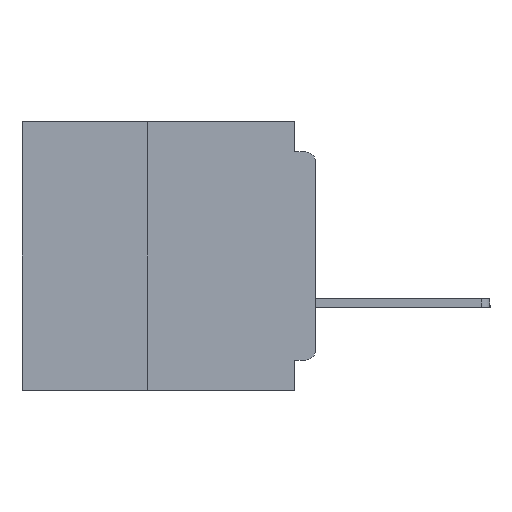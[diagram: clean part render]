
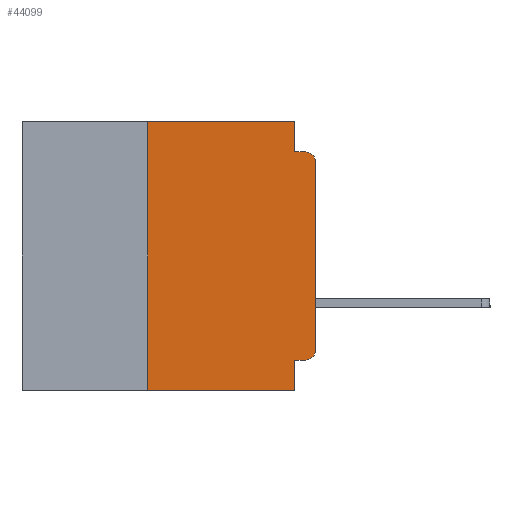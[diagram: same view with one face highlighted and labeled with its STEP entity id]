
A CAD part, left-side view. The second image highlights one B-rep face of the part: STEP entity #44099.
In plain terms, the highlighted planar face has unit normal (-1, 0, 0).
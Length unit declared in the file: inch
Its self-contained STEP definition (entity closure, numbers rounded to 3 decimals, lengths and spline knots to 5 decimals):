
#526 = LINE ( 'NONE', #22657, #59497 ) ;
#994 = VERTEX_POINT ( 'NONE', #20678 ) ;
#1742 = CARTESIAN_POINT ( 'NONE',  ( 0., 0.437, 0. ) ) ;
#2908 = EDGE_CURVE ( 'NONE', #36911, #27660, #33118, .T. ) ;
#2958 = LINE ( 'NONE', #53123, #18271 ) ;
#3637 = CARTESIAN_POINT ( 'NONE',  ( 0., 0.031, -0.4 ) ) ;
#4300 = CARTESIAN_POINT ( 'NONE',  ( 0., 0.031, 0. ) ) ;
#6065 = ORIENTED_EDGE ( 'NONE', *, *, #49792, .T. ) ;
#6183 = DIRECTION ( 'NONE',  ( 0., 0., -1. ) ) ;
#6405 = CIRCLE ( 'NONE', #38215, 0.015 ) ;
#6409 = PLANE ( 'NONE',  #52986 ) ;
#6523 = FACE_OUTER_BOUND ( 'NONE', #28270, .T. ) ;
#8288 = VECTOR ( 'NONE', #56010, 39.37008 ) ;
#8735 = DIRECTION ( 'NONE',  ( 0., -1., 0. ) ) ;
#8841 = LINE ( 'NONE', #49030, #32197 ) ;
#11990 = ORIENTED_EDGE ( 'NONE', *, *, #19523, .T. ) ;
#13692 = LINE ( 'NONE', #60333, #47957 ) ;
#14111 = DIRECTION ( 'NONE',  ( -1., 0., 0. ) ) ;
#14444 = VERTEX_POINT ( 'NONE', #48058 ) ;
#14611 = AXIS2_PLACEMENT_3D ( 'NONE', #42071, #14111, #46723 ) ;
#15791 = DIRECTION ( 'NONE',  ( 0., 0., -1. ) ) ;
#16769 = EDGE_CURVE ( 'NONE', #31690, #25327, #13692, .T. ) ;
#17154 = ORIENTED_EDGE ( 'NONE', *, *, #16769, .F. ) ;
#17900 = ORIENTED_EDGE ( 'NONE', *, *, #31625, .T. ) ;
#18271 = VECTOR ( 'NONE', #57808, 39.37008 ) ;
#18971 = VECTOR ( 'NONE', #6183, 39.37008 ) ;
#19523 = EDGE_CURVE ( 'NONE', #44456, #994, #24437, .T. ) ;
#20619 = DIRECTION ( 'NONE',  ( 0., 0., -1. ) ) ;
#20678 = CARTESIAN_POINT ( 'NONE',  ( 0., 0., -0.34 ) ) ;
#21519 = CARTESIAN_POINT ( 'NONE',  ( 0., 0., -0.355 ) ) ;
#21760 = LINE ( 'NONE', #25354, #57418 ) ;
#22657 = CARTESIAN_POINT ( 'NONE',  ( 0., 0., -0.045 ) ) ;
#22922 = VECTOR ( 'NONE', #58714, 39.37008 ) ;
#22996 = DIRECTION ( 'NONE',  ( 0., -1., 0. ) ) ;
#24437 = CIRCLE ( 'NONE', #14611, 0.015 ) ;
#24938 = EDGE_CURVE ( 'NONE', #25327, #28747, #31392, .T. ) ;
#25327 = VERTEX_POINT ( 'NONE', #4300 ) ;
#25354 = CARTESIAN_POINT ( 'NONE',  ( 0., 0.031, -0.4 ) ) ;
#25962 = DIRECTION ( 'NONE',  ( -1., 0., 0. ) ) ;
#27660 = VERTEX_POINT ( 'NONE', #3637 ) ;
#28270 = EDGE_LOOP ( 'NONE', ( #6065, #17900, #44654, #50144, #17154, #36712, #51407, #57345, #50468, #11990 ) ) ;
#28747 = VERTEX_POINT ( 'NONE', #30287 ) ;
#30287 = CARTESIAN_POINT ( 'NONE',  ( 0., 0.031, -0.045 ) ) ;
#31392 = LINE ( 'NONE', #38831, #18971 ) ;
#31576 = EDGE_CURVE ( 'NONE', #14444, #27660, #21760, .T. ) ;
#31625 = EDGE_CURVE ( 'NONE', #54610, #39142, #6405, .T. ) ;
#31690 = VERTEX_POINT ( 'NONE', #49705 ) ;
#32197 = VECTOR ( 'NONE', #48824, 39.37008 ) ;
#32480 = CARTESIAN_POINT ( 'NONE',  ( 0., 0.015, -0.045 ) ) ;
#33118 = LINE ( 'NONE', #42016, #8288 ) ;
#36712 = ORIENTED_EDGE ( 'NONE', *, *, #50391, .F. ) ;
#36911 = VERTEX_POINT ( 'NONE', #51762 ) ;
#38215 = AXIS2_PLACEMENT_3D ( 'NONE', #53772, #25962, #58422 ) ;
#38831 = CARTESIAN_POINT ( 'NONE',  ( 0., 0.031, 0. ) ) ;
#39142 = VERTEX_POINT ( 'NONE', #32480 ) ;
#42016 = CARTESIAN_POINT ( 'NONE',  ( 0., 0.437, -0.4 ) ) ;
#42071 = CARTESIAN_POINT ( 'NONE',  ( 0., 0.015, -0.34 ) ) ;
#43757 = DIRECTION ( 'NONE',  ( 1., 0., 0. ) ) ;
#44099 = ADVANCED_FACE ( 'NONE', ( #6523 ), #6409, .F. ) ;
#44456 = VERTEX_POINT ( 'NONE', #55244 ) ;
#44654 = ORIENTED_EDGE ( 'NONE', *, *, #46126, .F. ) ;
#45055 = CARTESIAN_POINT ( 'NONE',  ( 0., 0., -0.06 ) ) ;
#46126 = EDGE_CURVE ( 'NONE', #28747, #39142, #526, .T. ) ;
#46723 = DIRECTION ( 'NONE',  ( 0., 0., -1. ) ) ;
#47957 = VECTOR ( 'NONE', #22996, 39.37008 ) ;
#48058 = CARTESIAN_POINT ( 'NONE',  ( 0., 0.031, -0.355 ) ) ;
#48064 = EDGE_CURVE ( 'NONE', #44456, #14444, #50579, .T. ) ;
#48824 = DIRECTION ( 'NONE',  ( 0., 0., 1. ) ) ;
#49030 = CARTESIAN_POINT ( 'NONE',  ( 0., 0., 0. ) ) ;
#49705 = CARTESIAN_POINT ( 'NONE',  ( 0., 0.25, 0. ) ) ;
#49792 = EDGE_CURVE ( 'NONE', #994, #54610, #8841, .T. ) ;
#50144 = ORIENTED_EDGE ( 'NONE', *, *, #24938, .F. ) ;
#50391 = EDGE_CURVE ( 'NONE', #36911, #31690, #2958, .T. ) ;
#50468 = ORIENTED_EDGE ( 'NONE', *, *, #48064, .F. ) ;
#50579 = LINE ( 'NONE', #21519, #22922 ) ;
#51407 = ORIENTED_EDGE ( 'NONE', *, *, #2908, .T. ) ;
#51762 = CARTESIAN_POINT ( 'NONE',  ( 0., 0.25, -0.4 ) ) ;
#52986 = AXIS2_PLACEMENT_3D ( 'NONE', #1742, #43757, #15791 ) ;
#53123 = CARTESIAN_POINT ( 'NONE',  ( 0., 0.25, -0.4 ) ) ;
#53772 = CARTESIAN_POINT ( 'NONE',  ( 0., 0.015, -0.06 ) ) ;
#54610 = VERTEX_POINT ( 'NONE', #45055 ) ;
#55244 = CARTESIAN_POINT ( 'NONE',  ( 0., 0.015, -0.355 ) ) ;
#56010 = DIRECTION ( 'NONE',  ( 0., -1., 0. ) ) ;
#57345 = ORIENTED_EDGE ( 'NONE', *, *, #31576, .F. ) ;
#57418 = VECTOR ( 'NONE', #20619, 39.37008 ) ;
#57808 = DIRECTION ( 'NONE',  ( 0., 0., 1. ) ) ;
#58422 = DIRECTION ( 'NONE',  ( 0., 0., -1. ) ) ;
#58714 = DIRECTION ( 'NONE',  ( 0., 1., 0. ) ) ;
#59497 = VECTOR ( 'NONE', #8735, 39.37008 ) ;
#60333 = CARTESIAN_POINT ( 'NONE',  ( 0., 0.437, 0. ) ) ;
